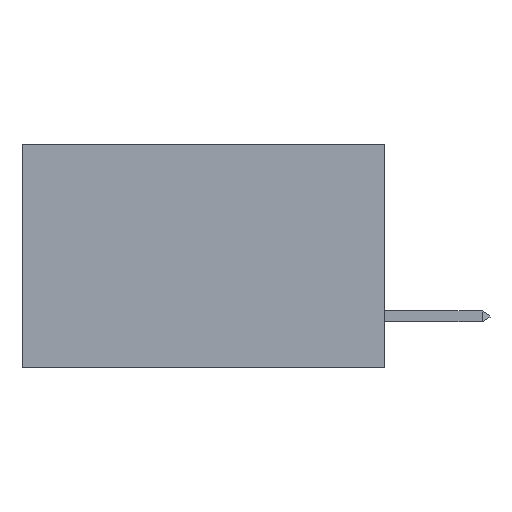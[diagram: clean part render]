
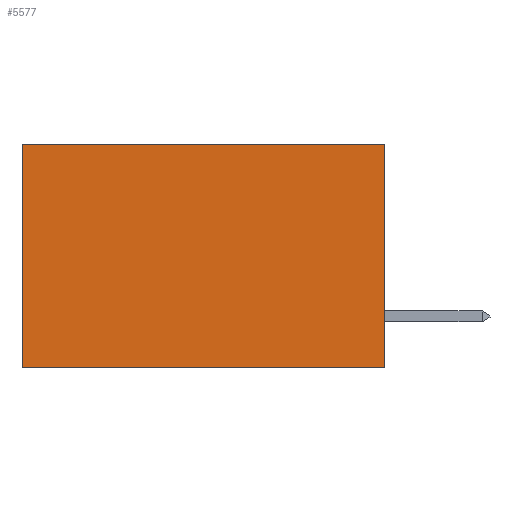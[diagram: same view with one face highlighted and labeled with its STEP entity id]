
A CAD part, left-side view. The second image highlights one B-rep face of the part: STEP entity #5577.
In plain terms, the highlighted planar face has unit normal (-1, 0, 0).
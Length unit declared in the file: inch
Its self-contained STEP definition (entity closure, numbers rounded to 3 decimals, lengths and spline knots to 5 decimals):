
#1456 = PLANE ( 'NONE',  #14384 ) ;
#1616 = LINE ( 'NONE', #10121, #8268 ) ;
#1698 = CARTESIAN_POINT ( 'NONE',  ( 0.2875, 0.6, -0.37 ) ) ;
#2018 = LINE ( 'NONE', #11476, #8217 ) ;
#2795 = LINE ( 'NONE', #3192, #6344 ) ;
#2900 = CARTESIAN_POINT ( 'NONE',  ( 0.2875, 0., 0. ) ) ;
#2918 = VECTOR ( 'NONE', #13108, 39.37008 ) ;
#2976 = VERTEX_POINT ( 'NONE', #4815 ) ;
#3192 = CARTESIAN_POINT ( 'NONE',  ( 0.2875, 0., 0. ) ) ;
#3233 = EDGE_CURVE ( 'NONE', #2976, #7283, #6464, .T. ) ;
#3607 = ORIENTED_EDGE ( 'NONE', *, *, #3233, .F. ) ;
#4186 = DIRECTION ( 'NONE',  ( 0., 0., -1. ) ) ;
#4665 = CARTESIAN_POINT ( 'NONE',  ( 0.2875, 0.6, 0. ) ) ;
#4815 = CARTESIAN_POINT ( 'NONE',  ( 0.2875, 0., 0. ) ) ;
#5478 = EDGE_CURVE ( 'NONE', #7975, #13409, #2018, .T. ) ;
#5505 = ORIENTED_EDGE ( 'NONE', *, *, #8584, .T. ) ;
#5577 = ADVANCED_FACE ( 'NONE', ( #7048 ), #1456, .F. ) ;
#5609 = DIRECTION ( 'NONE',  ( 1., 0., 0. ) ) ;
#6344 = VECTOR ( 'NONE', #12911, 39.37008 ) ;
#6464 = LINE ( 'NONE', #11748, #2918 ) ;
#7048 = FACE_OUTER_BOUND ( 'NONE', #13653, .T. ) ;
#7283 = VERTEX_POINT ( 'NONE', #14195 ) ;
#7876 = ORIENTED_EDGE ( 'NONE', *, *, #5478, .T. ) ;
#7975 = VERTEX_POINT ( 'NONE', #4665 ) ;
#8217 = VECTOR ( 'NONE', #4186, 39.37008 ) ;
#8268 = VECTOR ( 'NONE', #11222, 39.37008 ) ;
#8584 = EDGE_CURVE ( 'NONE', #2976, #7975, #2795, .T. ) ;
#10121 = CARTESIAN_POINT ( 'NONE',  ( 0.2875, 0., -0.37 ) ) ;
#11222 = DIRECTION ( 'NONE',  ( 0., 1., 0. ) ) ;
#11422 = EDGE_CURVE ( 'NONE', #7283, #13409, #1616, .T. ) ;
#11476 = CARTESIAN_POINT ( 'NONE',  ( 0.2875, 0.6, 0. ) ) ;
#11568 = ORIENTED_EDGE ( 'NONE', *, *, #11422, .F. ) ;
#11748 = CARTESIAN_POINT ( 'NONE',  ( 0.2875, 0., 0. ) ) ;
#12911 = DIRECTION ( 'NONE',  ( 0., 1., 0. ) ) ;
#13108 = DIRECTION ( 'NONE',  ( 0., 0., -1. ) ) ;
#13409 = VERTEX_POINT ( 'NONE', #1698 ) ;
#13653 = EDGE_LOOP ( 'NONE', ( #7876, #11568, #3607, #5505 ) ) ;
#13849 = DIRECTION ( 'NONE',  ( 0., 0., -1. ) ) ;
#14195 = CARTESIAN_POINT ( 'NONE',  ( 0.2875, 0., -0.37 ) ) ;
#14384 = AXIS2_PLACEMENT_3D ( 'NONE', #2900, #5609, #13849 ) ;
